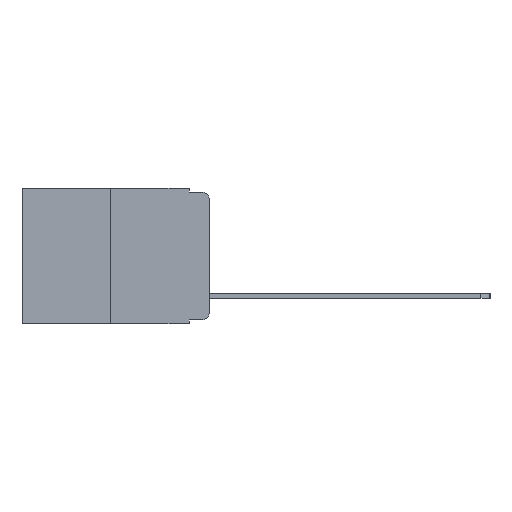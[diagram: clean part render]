
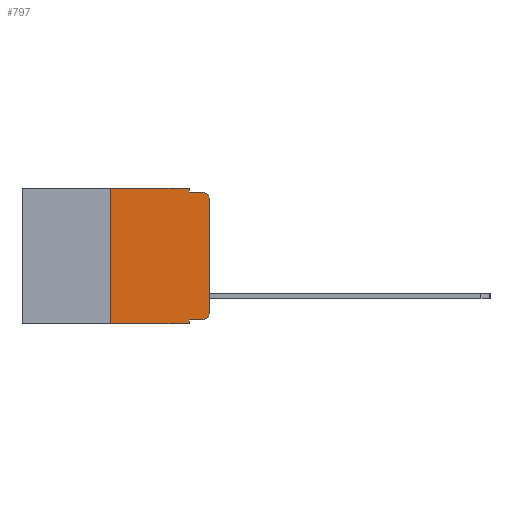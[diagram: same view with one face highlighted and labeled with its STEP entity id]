
A CAD part, left-side view. The second image highlights one B-rep face of the part: STEP entity #797.
In plain terms, the highlighted planar face has unit normal (-1, 0, 0).
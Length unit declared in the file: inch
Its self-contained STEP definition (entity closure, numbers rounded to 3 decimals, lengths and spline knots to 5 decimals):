
#733 = VERTEX_POINT ( 'NONE', #4609 ) ;
#797 = ADVANCED_FACE ( 'NONE', ( #10080 ), #16768, .F. ) ;
#890 = VECTOR ( 'NONE', #20669, 39.37008 ) ;
#1011 = DIRECTION ( 'NONE',  ( 0., -1., 0. ) ) ;
#1305 = EDGE_CURVE ( 'NONE', #20248, #3552, #19172, .T. ) ;
#1470 = LINE ( 'NONE', #11161, #890 ) ;
#1950 = VERTEX_POINT ( 'NONE', #4369 ) ;
#2722 = LINE ( 'NONE', #21131, #19769 ) ;
#2874 = EDGE_LOOP ( 'NONE', ( #14199, #14523, #15343, #15567, #15752, #16764, #20089, #21182, #3045, #11329 ) ) ;
#3045 = ORIENTED_EDGE ( 'NONE', *, *, #3120, .T. ) ;
#3120 = EDGE_CURVE ( 'NONE', #5428, #20248, #15661, .T. ) ;
#3281 = DIRECTION ( 'NONE',  ( 0., 0., -1. ) ) ;
#3552 = VERTEX_POINT ( 'NONE', #21500 ) ;
#3648 = LINE ( 'NONE', #5750, #16502 ) ;
#4302 = DIRECTION ( 'NONE',  ( 0., -1., 0. ) ) ;
#4324 = EDGE_CURVE ( 'NONE', #17355, #9637, #1470, .T. ) ;
#4369 = CARTESIAN_POINT ( 'NONE',  ( 0., 0.25, 0. ) ) ;
#4394 = EDGE_CURVE ( 'NONE', #1950, #17355, #20804, .T. ) ;
#4430 = EDGE_CURVE ( 'NONE', #3552, #733, #6885, .T. ) ;
#4609 = CARTESIAN_POINT ( 'NONE',  ( 0., 0., -0.03 ) ) ;
#5133 = LINE ( 'NONE', #13473, #13080 ) ;
#5428 = VERTEX_POINT ( 'NONE', #18856 ) ;
#5750 = CARTESIAN_POINT ( 'NONE',  ( 0., 0.051, -0.01 ) ) ;
#6686 = VECTOR ( 'NONE', #16624, 39.37008 ) ;
#6789 = VECTOR ( 'NONE', #4302, 39.37008 ) ;
#6804 = DIRECTION ( 'NONE',  ( 0., 0., -1. ) ) ;
#6885 = LINE ( 'NONE', #9780, #19856 ) ;
#6993 = AXIS2_PLACEMENT_3D ( 'NONE', #18015, #8373, #6804 ) ;
#7190 = AXIS2_PLACEMENT_3D ( 'NONE', #17197, #7272, #18736 ) ;
#7200 = LINE ( 'NONE', #15047, #6686 ) ;
#7272 = DIRECTION ( 'NONE',  ( -1., 0., 0. ) ) ;
#7458 = DIRECTION ( 'NONE',  ( 0., -1., 0. ) ) ;
#8373 = DIRECTION ( 'NONE',  ( -1., 0., 0. ) ) ;
#9030 = VECTOR ( 'NONE', #1011, 39.37008 ) ;
#9044 = EDGE_CURVE ( 'NONE', #9637, #17365, #3648, .T. ) ;
#9637 = VERTEX_POINT ( 'NONE', #20181 ) ;
#9780 = CARTESIAN_POINT ( 'NONE',  ( 0., 0., 0. ) ) ;
#9979 = CARTESIAN_POINT ( 'NONE',  ( 0., 0.051, 0. ) ) ;
#10080 = FACE_OUTER_BOUND ( 'NONE', #2874, .T. ) ;
#11161 = CARTESIAN_POINT ( 'NONE',  ( 0., 0.051, 0. ) ) ;
#11309 = EDGE_CURVE ( 'NONE', #14909, #1950, #2722, .T. ) ;
#11329 = ORIENTED_EDGE ( 'NONE', *, *, #1305, .T. ) ;
#12979 = CIRCLE ( 'NONE', #7190, 0.02 ) ;
#13080 = VECTOR ( 'NONE', #3281, 39.37008 ) ;
#13473 = CARTESIAN_POINT ( 'NONE',  ( 0., 0.051, 0. ) ) ;
#14199 = ORIENTED_EDGE ( 'NONE', *, *, #4430, .T. ) ;
#14441 = CARTESIAN_POINT ( 'NONE',  ( 0., 0.051, -0.333 ) ) ;
#14523 = ORIENTED_EDGE ( 'NONE', *, *, #14655, .T. ) ;
#14655 = EDGE_CURVE ( 'NONE', #733, #17365, #12979, .T. ) ;
#14909 = VERTEX_POINT ( 'NONE', #17745 ) ;
#14980 = CARTESIAN_POINT ( 'NONE',  ( 0., 0.02, -0.01 ) ) ;
#15047 = CARTESIAN_POINT ( 'NONE',  ( 0., 0.473, -0.343 ) ) ;
#15343 = ORIENTED_EDGE ( 'NONE', *, *, #9044, .F. ) ;
#15567 = ORIENTED_EDGE ( 'NONE', *, *, #4324, .F. ) ;
#15661 = LINE ( 'NONE', #14441, #6789 ) ;
#15752 = ORIENTED_EDGE ( 'NONE', *, *, #4394, .F. ) ;
#15911 = CARTESIAN_POINT ( 'NONE',  ( 0., 0.051, -0.343 ) ) ;
#16502 = VECTOR ( 'NONE', #7458, 39.37008 ) ;
#16572 = DIRECTION ( 'NONE',  ( 0., 0., 1. ) ) ;
#16624 = DIRECTION ( 'NONE',  ( 0., -1., 0. ) ) ;
#16649 = DIRECTION ( 'NONE',  ( 1., 0., 0. ) ) ;
#16764 = ORIENTED_EDGE ( 'NONE', *, *, #11309, .F. ) ;
#16768 = PLANE ( 'NONE',  #17905 ) ;
#17197 = CARTESIAN_POINT ( 'NONE',  ( 0., 0.02, -0.03 ) ) ;
#17355 = VERTEX_POINT ( 'NONE', #9979 ) ;
#17365 = VERTEX_POINT ( 'NONE', #14980 ) ;
#17441 = EDGE_CURVE ( 'NONE', #5428, #21111, #5133, .T. ) ;
#17745 = CARTESIAN_POINT ( 'NONE',  ( 0., 0.25, -0.343 ) ) ;
#17905 = AXIS2_PLACEMENT_3D ( 'NONE', #18991, #16649, #19176 ) ;
#18015 = CARTESIAN_POINT ( 'NONE',  ( 0., 0.02, -0.313 ) ) ;
#18736 = DIRECTION ( 'NONE',  ( 0., 0., -1. ) ) ;
#18856 = CARTESIAN_POINT ( 'NONE',  ( 0., 0.051, -0.333 ) ) ;
#18991 = CARTESIAN_POINT ( 'NONE',  ( 0., 0.473, 0. ) ) ;
#19172 = CIRCLE ( 'NONE', #6993, 0.02 ) ;
#19176 = DIRECTION ( 'NONE',  ( 0., 0., -1. ) ) ;
#19769 = VECTOR ( 'NONE', #16572, 39.37008 ) ;
#19856 = VECTOR ( 'NONE', #20943, 39.37008 ) ;
#20089 = ORIENTED_EDGE ( 'NONE', *, *, #20733, .T. ) ;
#20181 = CARTESIAN_POINT ( 'NONE',  ( 0., 0.051, -0.01 ) ) ;
#20182 = CARTESIAN_POINT ( 'NONE',  ( 0., 0.02, -0.333 ) ) ;
#20248 = VERTEX_POINT ( 'NONE', #20182 ) ;
#20669 = DIRECTION ( 'NONE',  ( 0., 0., -1. ) ) ;
#20733 = EDGE_CURVE ( 'NONE', #14909, #21111, #7200, .T. ) ;
#20792 = CARTESIAN_POINT ( 'NONE',  ( 0., 0.473, 0. ) ) ;
#20804 = LINE ( 'NONE', #20792, #9030 ) ;
#20943 = DIRECTION ( 'NONE',  ( 0., 0., 1. ) ) ;
#21111 = VERTEX_POINT ( 'NONE', #15911 ) ;
#21131 = CARTESIAN_POINT ( 'NONE',  ( 0., 0.25, 0. ) ) ;
#21182 = ORIENTED_EDGE ( 'NONE', *, *, #17441, .F. ) ;
#21500 = CARTESIAN_POINT ( 'NONE',  ( 0., 0., -0.313 ) ) ;
